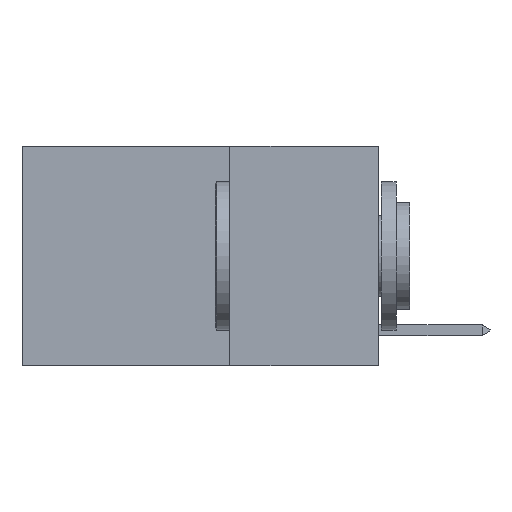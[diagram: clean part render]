
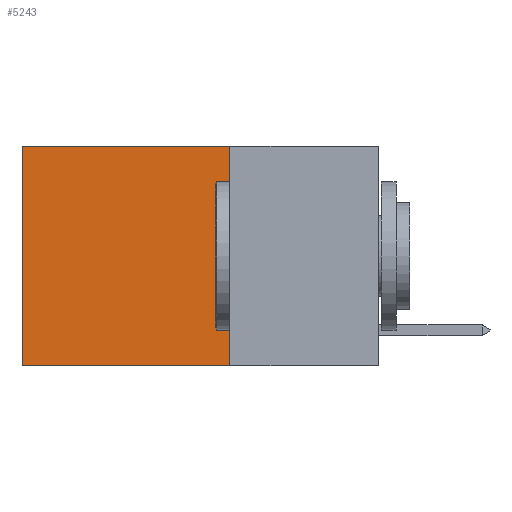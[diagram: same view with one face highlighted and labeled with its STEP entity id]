
A CAD part, left-side view. The second image highlights one B-rep face of the part: STEP entity #5243.
In plain terms, the highlighted planar face has unit normal (-1, 0, 0).
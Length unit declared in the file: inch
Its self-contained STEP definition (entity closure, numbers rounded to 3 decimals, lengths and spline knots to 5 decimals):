
#5 = DIRECTION ( 'NONE',  ( 0., 1., 0. ) ) ;
#129 = CARTESIAN_POINT ( 'NONE',  ( 0.2625, 0.25, -0.37 ) ) ;
#455 = CARTESIAN_POINT ( 'NONE',  ( 0.2625, 0.25, 0. ) ) ;
#907 = LINE ( 'NONE', #7700, #9861 ) ;
#940 = AXIS2_PLACEMENT_3D ( 'NONE', #455, #3330, #4046 ) ;
#1179 = PLANE ( 'NONE',  #940 ) ;
#1385 = DIRECTION ( 'NONE',  ( 0., 0., -1. ) ) ;
#1555 = ORIENTED_EDGE ( 'NONE', *, *, #9714, .T. ) ;
#2963 = FACE_OUTER_BOUND ( 'NONE', #9738, .T. ) ;
#3280 = CARTESIAN_POINT ( 'NONE',  ( 0.2625, 0.6, 0. ) ) ;
#3330 = DIRECTION ( 'NONE',  ( 1., 0., 0. ) ) ;
#3376 = DIRECTION ( 'NONE',  ( 0., 1., 0. ) ) ;
#3615 = VECTOR ( 'NONE', #5, 39.37008 ) ;
#3892 = LINE ( 'NONE', #6454, #3615 ) ;
#4046 = DIRECTION ( 'NONE',  ( 0., 0., -1. ) ) ;
#4194 = CARTESIAN_POINT ( 'NONE',  ( 0.2625, 0.25, 0. ) ) ;
#4251 = CARTESIAN_POINT ( 'NONE',  ( 0.2625, 0.25, -0.37 ) ) ;
#4278 = EDGE_CURVE ( 'NONE', #7110, #9965, #4663, .T. ) ;
#4404 = VECTOR ( 'NONE', #3376, 39.37008 ) ;
#4663 = LINE ( 'NONE', #4251, #4404 ) ;
#5243 = ADVANCED_FACE ( 'NONE', ( #2963 ), #1179, .F. ) ;
#5274 = VERTEX_POINT ( 'NONE', #4194 ) ;
#5277 = VERTEX_POINT ( 'NONE', #3280 ) ;
#5952 = ORIENTED_EDGE ( 'NONE', *, *, #4278, .F. ) ;
#6454 = CARTESIAN_POINT ( 'NONE',  ( 0.2625, 0.25, 0. ) ) ;
#7110 = VERTEX_POINT ( 'NONE', #129 ) ;
#7700 = CARTESIAN_POINT ( 'NONE',  ( 0.2625, 0.6, 0. ) ) ;
#7894 = CARTESIAN_POINT ( 'NONE',  ( 0.2625, 0.6, -0.37 ) ) ;
#8576 = EDGE_CURVE ( 'NONE', #5277, #9965, #907, .T. ) ;
#8838 = LINE ( 'NONE', #9050, #10333 ) ;
#8844 = ORIENTED_EDGE ( 'NONE', *, *, #8576, .T. ) ;
#8958 = EDGE_CURVE ( 'NONE', #5274, #7110, #8838, .T. ) ;
#9050 = CARTESIAN_POINT ( 'NONE',  ( 0.2625, 0.25, 0. ) ) ;
#9116 = DIRECTION ( 'NONE',  ( 0., 0., -1. ) ) ;
#9335 = ORIENTED_EDGE ( 'NONE', *, *, #8958, .F. ) ;
#9714 = EDGE_CURVE ( 'NONE', #5274, #5277, #3892, .T. ) ;
#9738 = EDGE_LOOP ( 'NONE', ( #8844, #5952, #9335, #1555 ) ) ;
#9861 = VECTOR ( 'NONE', #1385, 39.37008 ) ;
#9965 = VERTEX_POINT ( 'NONE', #7894 ) ;
#10333 = VECTOR ( 'NONE', #9116, 39.37008 ) ;
